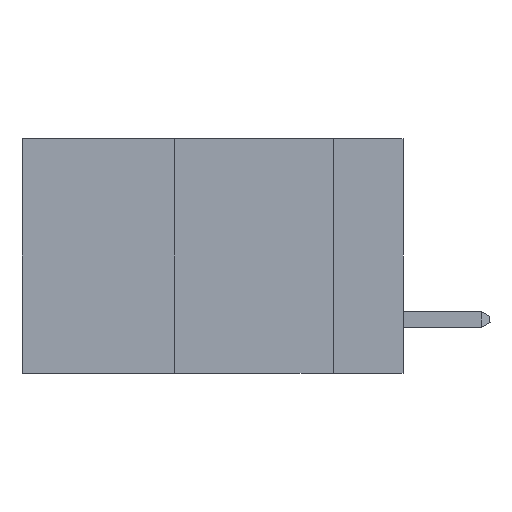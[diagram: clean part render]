
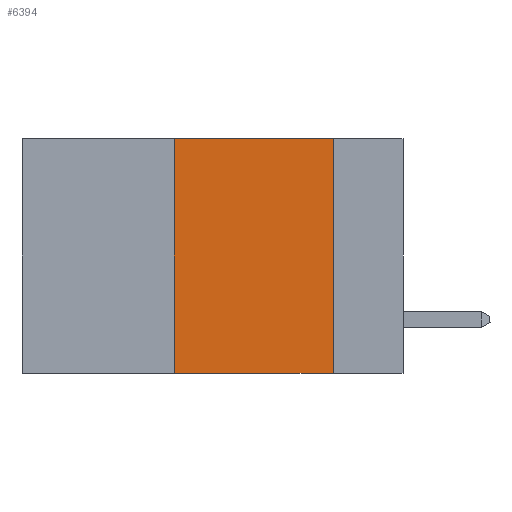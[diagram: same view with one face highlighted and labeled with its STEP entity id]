
A CAD part, left-side view. The second image highlights one B-rep face of the part: STEP entity #6394.
In plain terms, the highlighted planar face has unit normal (-1, 0, 0).
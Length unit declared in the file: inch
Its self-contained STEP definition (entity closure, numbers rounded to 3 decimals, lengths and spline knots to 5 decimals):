
#224 = LINE ( 'NONE', #7222, #2033 ) ;
#622 = LINE ( 'NONE', #2774, #3534 ) ;
#677 = DIRECTION ( 'NONE',  ( 0., 0., 1. ) ) ;
#1022 = ORIENTED_EDGE ( 'NONE', *, *, #3397, .F. ) ;
#1250 = LINE ( 'NONE', #5043, #6874 ) ;
#1949 = ORIENTED_EDGE ( 'NONE', *, *, #6918, .F. ) ;
#2033 = VECTOR ( 'NONE', #5153, 39.37008 ) ;
#2125 = VECTOR ( 'NONE', #3370, 39.37008 ) ;
#2134 = DIRECTION ( 'NONE',  ( 1., 0., 0. ) ) ;
#2145 = CARTESIAN_POINT ( 'NONE',  ( 0., 0.36, 0. ) ) ;
#2342 = CARTESIAN_POINT ( 'NONE',  ( 0., 0.11, 0. ) ) ;
#2405 = VERTEX_POINT ( 'NONE', #7173 ) ;
#2712 = PLANE ( 'NONE',  #7580 ) ;
#2774 = CARTESIAN_POINT ( 'NONE',  ( 0., 0.36, 0. ) ) ;
#2928 = EDGE_CURVE ( 'NONE', #2405, #3210, #224, .T. ) ;
#3210 = VERTEX_POINT ( 'NONE', #8043 ) ;
#3370 = DIRECTION ( 'NONE',  ( 0., -1., 0. ) ) ;
#3397 = EDGE_CURVE ( 'NONE', #2405, #5649, #622, .T. ) ;
#3534 = VECTOR ( 'NONE', #677, 39.37008 ) ;
#4549 = EDGE_LOOP ( 'NONE', ( #4934, #1949, #1022, #5978 ) ) ;
#4782 = CARTESIAN_POINT ( 'NONE',  ( 0., 0.6, 0. ) ) ;
#4788 = VERTEX_POINT ( 'NONE', #2342 ) ;
#4934 = ORIENTED_EDGE ( 'NONE', *, *, #7706, .F. ) ;
#5043 = CARTESIAN_POINT ( 'NONE',  ( 0., 0.11, 0. ) ) ;
#5153 = DIRECTION ( 'NONE',  ( 0., -1., 0. ) ) ;
#5464 = DIRECTION ( 'NONE',  ( 0., 0., -1. ) ) ;
#5649 = VERTEX_POINT ( 'NONE', #2145 ) ;
#5978 = ORIENTED_EDGE ( 'NONE', *, *, #2928, .T. ) ;
#6394 = ADVANCED_FACE ( 'NONE', ( #6461 ), #2712, .F. ) ;
#6461 = FACE_OUTER_BOUND ( 'NONE', #4549, .T. ) ;
#6874 = VECTOR ( 'NONE', #8439, 39.37008 ) ;
#6918 = EDGE_CURVE ( 'NONE', #5649, #4788, #8576, .T. ) ;
#7173 = CARTESIAN_POINT ( 'NONE',  ( 0., 0.36, -0.37 ) ) ;
#7222 = CARTESIAN_POINT ( 'NONE',  ( 0., 0.6, -0.37 ) ) ;
#7456 = CARTESIAN_POINT ( 'NONE',  ( 0., 0.6, 0. ) ) ;
#7580 = AXIS2_PLACEMENT_3D ( 'NONE', #4782, #2134, #5464 ) ;
#7706 = EDGE_CURVE ( 'NONE', #4788, #3210, #1250, .T. ) ;
#8043 = CARTESIAN_POINT ( 'NONE',  ( 0., 0.11, -0.37 ) ) ;
#8439 = DIRECTION ( 'NONE',  ( 0., 0., -1. ) ) ;
#8576 = LINE ( 'NONE', #7456, #2125 ) ;
